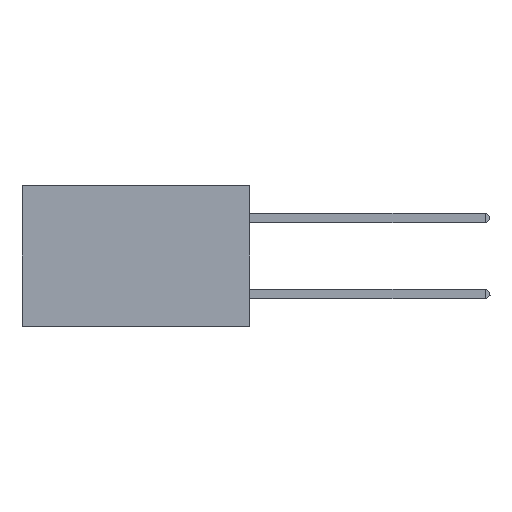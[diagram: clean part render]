
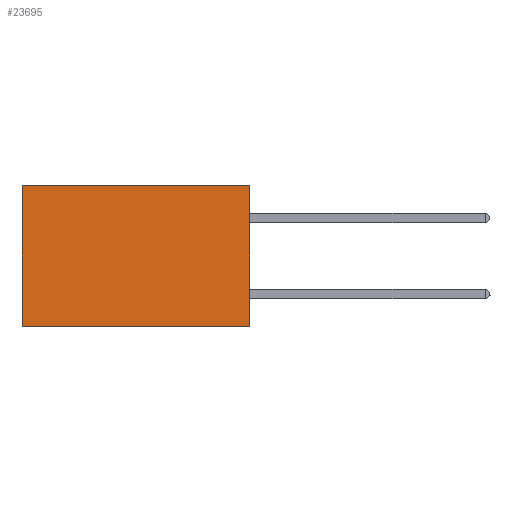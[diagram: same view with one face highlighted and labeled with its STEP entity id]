
A CAD part, left-side view. The second image highlights one B-rep face of the part: STEP entity #23695.
In plain terms, the highlighted planar face has unit normal (-1, 0, 0).
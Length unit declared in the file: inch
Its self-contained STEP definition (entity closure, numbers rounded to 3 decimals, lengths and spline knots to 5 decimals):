
#2271 = DIRECTION ( 'NONE',  ( 0., 0., -1. ) ) ;
#3363 = CARTESIAN_POINT ( 'NONE',  ( 0.2875, 0., 0. ) ) ;
#7442 = DIRECTION ( 'NONE',  ( 0., 1., 0. ) ) ;
#9088 = CARTESIAN_POINT ( 'NONE',  ( 0.2875, 0., 0. ) ) ;
#11869 = VERTEX_POINT ( 'NONE', #23399 ) ;
#14287 = VECTOR ( 'NONE', #2271, 39.37008 ) ;
#14678 = ORIENTED_EDGE ( 'NONE', *, *, #21009, .T. ) ;
#15958 = ORIENTED_EDGE ( 'NONE', *, *, #27629, .F. ) ;
#16357 = VECTOR ( 'NONE', #7442, 39.37008 ) ;
#17032 = CARTESIAN_POINT ( 'NONE',  ( 0.2875, 0.6, 0. ) ) ;
#17074 = EDGE_CURVE ( 'NONE', #18559, #26211, #17439, .T. ) ;
#17439 = LINE ( 'NONE', #3363, #23864 ) ;
#17475 = AXIS2_PLACEMENT_3D ( 'NONE', #39409, #35935, #23445 ) ;
#18174 = LINE ( 'NONE', #17032, #30549 ) ;
#18559 = VERTEX_POINT ( 'NONE', #26229 ) ;
#20286 = PLANE ( 'NONE',  #17475 ) ;
#20406 = CARTESIAN_POINT ( 'NONE',  ( 0.2875, 0., -0.37 ) ) ;
#20763 = LINE ( 'NONE', #9088, #14287 ) ;
#21009 = EDGE_CURVE ( 'NONE', #26211, #21268, #18174, .T. ) ;
#21268 = VERTEX_POINT ( 'NONE', #39923 ) ;
#23399 = CARTESIAN_POINT ( 'NONE',  ( 0.2875, 0., -0.37 ) ) ;
#23445 = DIRECTION ( 'NONE',  ( 0., 0., -1. ) ) ;
#23695 = ADVANCED_FACE ( 'NONE', ( #23872 ), #20286, .F. ) ;
#23864 = VECTOR ( 'NONE', #25762, 39.37008 ) ;
#23872 = FACE_OUTER_BOUND ( 'NONE', #30550, .T. ) ;
#25762 = DIRECTION ( 'NONE',  ( 0., 1., 0. ) ) ;
#26211 = VERTEX_POINT ( 'NONE', #28060 ) ;
#26229 = CARTESIAN_POINT ( 'NONE',  ( 0.2875, 0., 0. ) ) ;
#27629 = EDGE_CURVE ( 'NONE', #18559, #11869, #20763, .T. ) ;
#28060 = CARTESIAN_POINT ( 'NONE',  ( 0.2875, 0.6, 0. ) ) ;
#29365 = DIRECTION ( 'NONE',  ( 0., 0., -1. ) ) ;
#30376 = ORIENTED_EDGE ( 'NONE', *, *, #17074, .T. ) ;
#30549 = VECTOR ( 'NONE', #29365, 39.37008 ) ;
#30550 = EDGE_LOOP ( 'NONE', ( #14678, #39835, #15958, #30376 ) ) ;
#32374 = EDGE_CURVE ( 'NONE', #11869, #21268, #36227, .T. ) ;
#35935 = DIRECTION ( 'NONE',  ( 1., 0., 0. ) ) ;
#36227 = LINE ( 'NONE', #20406, #16357 ) ;
#39409 = CARTESIAN_POINT ( 'NONE',  ( 0.2875, 0., 0. ) ) ;
#39835 = ORIENTED_EDGE ( 'NONE', *, *, #32374, .F. ) ;
#39923 = CARTESIAN_POINT ( 'NONE',  ( 0.2875, 0.6, -0.37 ) ) ;
